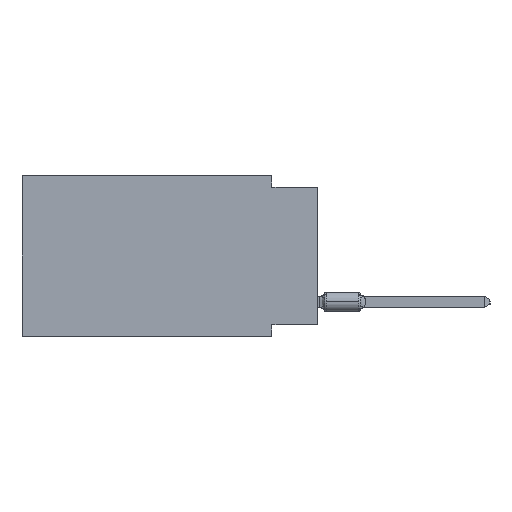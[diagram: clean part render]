
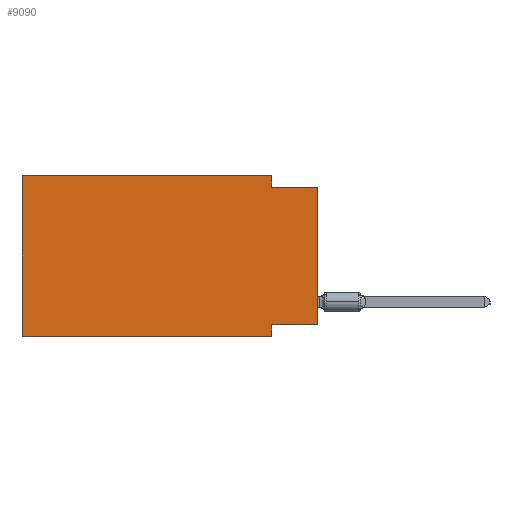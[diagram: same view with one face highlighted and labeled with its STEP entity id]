
A CAD part, left-side view. The second image highlights one B-rep face of the part: STEP entity #9090.
In plain terms, the highlighted planar face has unit normal (-1, 0, 0).
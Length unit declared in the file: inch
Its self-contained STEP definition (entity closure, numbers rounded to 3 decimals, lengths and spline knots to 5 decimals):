
#981 = VECTOR ( 'NONE', #84049, 39.37008 ) ;
#1381 = DIRECTION ( 'NONE',  ( 0., 0., 1. ) ) ;
#2313 = CARTESIAN_POINT ( 'NONE',  ( 0., 0.645, -0.35 ) ) ;
#2810 = ORIENTED_EDGE ( 'NONE', *, *, #36806, .F. ) ;
#3200 = DIRECTION ( 'NONE',  ( 0., 0., 1. ) ) ;
#3421 = EDGE_CURVE ( 'NONE', #91434, #65506, #103497, .T. ) ;
#3823 = VECTOR ( 'NONE', #76731, 39.37008 ) ;
#5087 = EDGE_CURVE ( 'NONE', #106299, #65506, #96845, .T. ) ;
#7744 = LINE ( 'NONE', #40808, #39179 ) ;
#7901 = CARTESIAN_POINT ( 'NONE',  ( 0., 0., 0. ) ) ;
#9090 = ADVANCED_FACE ( 'NONE', ( #89164 ), #88636, .F. ) ;
#10641 = LINE ( 'NONE', #79842, #58274 ) ;
#12647 = CARTESIAN_POINT ( 'NONE',  ( 0., 0.645, 0. ) ) ;
#13262 = CARTESIAN_POINT ( 'NONE',  ( 0., 0., -0.325 ) ) ;
#14704 = VECTOR ( 'NONE', #23103, 39.37008 ) ;
#17109 = ORIENTED_EDGE ( 'NONE', *, *, #5087, .F. ) ;
#17149 = EDGE_LOOP ( 'NONE', ( #78368, #18985, #93668, #98547, #32201, #81507, #17109, #2810 ) ) ;
#17351 = VECTOR ( 'NONE', #79638, 39.37008 ) ;
#18985 = ORIENTED_EDGE ( 'NONE', *, *, #49183, .F. ) ;
#23103 = DIRECTION ( 'NONE',  ( 0., 0., -1. ) ) ;
#25105 = VECTOR ( 'NONE', #1381, 39.37008 ) ;
#26464 = VERTEX_POINT ( 'NONE', #67135 ) ;
#31777 = CARTESIAN_POINT ( 'NONE',  ( 0., 0.1, -0.35 ) ) ;
#32201 = ORIENTED_EDGE ( 'NONE', *, *, #54609, .F. ) ;
#32234 = CARTESIAN_POINT ( 'NONE',  ( 0., 0.645, 0. ) ) ;
#33229 = DIRECTION ( 'NONE',  ( 0., -1., 0. ) ) ;
#36806 = EDGE_CURVE ( 'NONE', #26464, #106299, #37658, .T. ) ;
#37658 = LINE ( 'NONE', #13262, #3823 ) ;
#38612 = DIRECTION ( 'NONE',  ( 0., -1., 0. ) ) ;
#39179 = VECTOR ( 'NONE', #33229, 39.37008 ) ;
#40808 = CARTESIAN_POINT ( 'NONE',  ( 0., 0., -0.025 ) ) ;
#49183 = EDGE_CURVE ( 'NONE', #50812, #66514, #7744, .T. ) ;
#50812 = VERTEX_POINT ( 'NONE', #102652 ) ;
#54609 = EDGE_CURVE ( 'NONE', #91434, #88748, #77491, .T. ) ;
#58274 = VECTOR ( 'NONE', #38612, 39.37008 ) ;
#62388 = EDGE_CURVE ( 'NONE', #105070, #50812, #100306, .T. ) ;
#62969 = AXIS2_PLACEMENT_3D ( 'NONE', #32234, #98918, #89711 ) ;
#63532 = EDGE_CURVE ( 'NONE', #88748, #105070, #10641, .T. ) ;
#65506 = VERTEX_POINT ( 'NONE', #67759 ) ;
#66514 = VERTEX_POINT ( 'NONE', #73225 ) ;
#67135 = CARTESIAN_POINT ( 'NONE',  ( 0., 0., -0.325 ) ) ;
#67759 = CARTESIAN_POINT ( 'NONE',  ( 0., 0.1, -0.35 ) ) ;
#73225 = CARTESIAN_POINT ( 'NONE',  ( 0., 0., -0.025 ) ) ;
#76731 = DIRECTION ( 'NONE',  ( 0., 1., 0. ) ) ;
#77491 = LINE ( 'NONE', #78548, #102824 ) ;
#78368 = ORIENTED_EDGE ( 'NONE', *, *, #97113, .T. ) ;
#78548 = CARTESIAN_POINT ( 'NONE',  ( 0., 0.645, 0. ) ) ;
#79106 = CARTESIAN_POINT ( 'NONE',  ( 0., 0.645, -0.35 ) ) ;
#79638 = DIRECTION ( 'NONE',  ( 0., -1., 0. ) ) ;
#79842 = CARTESIAN_POINT ( 'NONE',  ( 0., 0.645, 0. ) ) ;
#81507 = ORIENTED_EDGE ( 'NONE', *, *, #3421, .T. ) ;
#83518 = CARTESIAN_POINT ( 'NONE',  ( 0., 0.1, 0. ) ) ;
#84049 = DIRECTION ( 'NONE',  ( 0., 0., -1. ) ) ;
#85765 = CARTESIAN_POINT ( 'NONE',  ( 0., 0.1, 0. ) ) ;
#88636 = PLANE ( 'NONE',  #62969 ) ;
#88748 = VERTEX_POINT ( 'NONE', #12647 ) ;
#89164 = FACE_OUTER_BOUND ( 'NONE', #17149, .T. ) ;
#89711 = DIRECTION ( 'NONE',  ( 0., 0., -1. ) ) ;
#91434 = VERTEX_POINT ( 'NONE', #2313 ) ;
#92445 = LINE ( 'NONE', #7901, #25105 ) ;
#93668 = ORIENTED_EDGE ( 'NONE', *, *, #62388, .F. ) ;
#96845 = LINE ( 'NONE', #31777, #14704 ) ;
#97113 = EDGE_CURVE ( 'NONE', #26464, #66514, #92445, .T. ) ;
#98547 = ORIENTED_EDGE ( 'NONE', *, *, #63532, .F. ) ;
#98918 = DIRECTION ( 'NONE',  ( 1., 0., 0. ) ) ;
#100306 = LINE ( 'NONE', #83518, #981 ) ;
#100525 = CARTESIAN_POINT ( 'NONE',  ( 0., 0.1, -0.325 ) ) ;
#102652 = CARTESIAN_POINT ( 'NONE',  ( 0., 0.1, -0.025 ) ) ;
#102824 = VECTOR ( 'NONE', #3200, 39.37008 ) ;
#103497 = LINE ( 'NONE', #79106, #17351 ) ;
#105070 = VERTEX_POINT ( 'NONE', #85765 ) ;
#106299 = VERTEX_POINT ( 'NONE', #100525 ) ;
